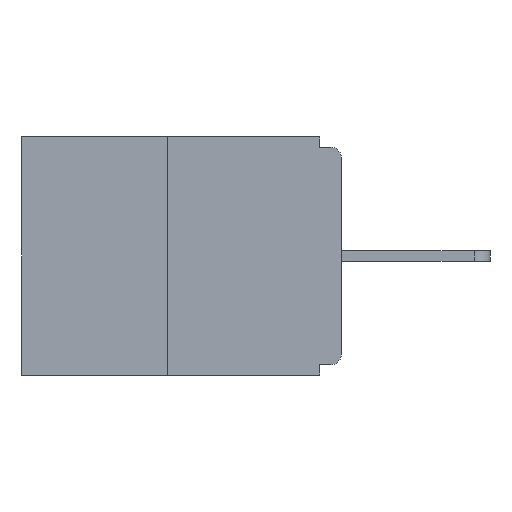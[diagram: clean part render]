
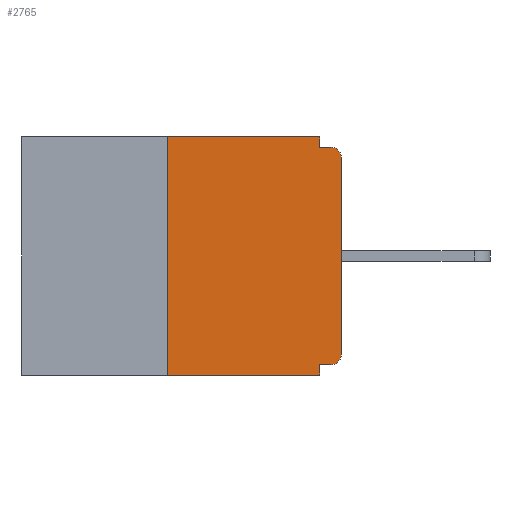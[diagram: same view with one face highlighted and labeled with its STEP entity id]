
A CAD part, left-side view. The second image highlights one B-rep face of the part: STEP entity #2765.
In plain terms, the highlighted planar face has unit normal (-1, 0, 0).
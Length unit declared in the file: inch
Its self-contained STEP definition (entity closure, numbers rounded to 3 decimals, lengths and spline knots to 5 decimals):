
#239 = EDGE_CURVE ( 'NONE', #16663, #10309, #5698, .T. ) ;
#665 = LINE ( 'NONE', #3332, #12376 ) ;
#744 = DIRECTION ( 'NONE',  ( 0., 1., 0. ) ) ;
#1418 = CARTESIAN_POINT ( 'NONE',  ( 0., 0.015, -0.015 ) ) ;
#1787 = DIRECTION ( 'NONE',  ( 0., -1., 0. ) ) ;
#1801 = ORIENTED_EDGE ( 'NONE', *, *, #16502, .F. ) ;
#2765 = ADVANCED_FACE ( 'NONE', ( #12053 ), #13118, .F. ) ;
#3188 = CARTESIAN_POINT ( 'NONE',  ( 0., 0., -0.015 ) ) ;
#3332 = CARTESIAN_POINT ( 'NONE',  ( 0., 0., 0. ) ) ;
#3457 = ORIENTED_EDGE ( 'NONE', *, *, #5095, .T. ) ;
#3521 = LINE ( 'NONE', #13514, #7980 ) ;
#3758 = CARTESIAN_POINT ( 'NONE',  ( 0., 0.46, -0.343 ) ) ;
#4011 = CARTESIAN_POINT ( 'NONE',  ( 0., 0.031, -0.343 ) ) ;
#4619 = ORIENTED_EDGE ( 'NONE', *, *, #11678, .F. ) ;
#4798 = CARTESIAN_POINT ( 'NONE',  ( 0., 0.46, 0. ) ) ;
#5000 = CARTESIAN_POINT ( 'NONE',  ( 0., 0., -0.313 ) ) ;
#5095 = EDGE_CURVE ( 'NONE', #15963, #8422, #14659, .T. ) ;
#5176 = DIRECTION ( 'NONE',  ( 0., 0., -1. ) ) ;
#5457 = EDGE_LOOP ( 'NONE', ( #1801, #9594, #7517, #4619, #17503, #3457, #9910, #11811, #14829, #15544 ) ) ;
#5698 = LINE ( 'NONE', #3758, #15821 ) ;
#5871 = EDGE_CURVE ( 'NONE', #8422, #12729, #665, .T. ) ;
#5959 = VECTOR ( 'NONE', #6125, 39.37008 ) ;
#6125 = DIRECTION ( 'NONE',  ( 0., -1., 0. ) ) ;
#6165 = DIRECTION ( 'NONE',  ( 1., 0., 0. ) ) ;
#6712 = AXIS2_PLACEMENT_3D ( 'NONE', #4798, #6165, #13174 ) ;
#6737 = VERTEX_POINT ( 'NONE', #17194 ) ;
#6806 = DIRECTION ( 'NONE',  ( -1., 0., 0. ) ) ;
#7517 = ORIENTED_EDGE ( 'NONE', *, *, #239, .T. ) ;
#7595 = CARTESIAN_POINT ( 'NONE',  ( 0., 0.015, -0.313 ) ) ;
#7692 = CARTESIAN_POINT ( 'NONE',  ( 0., 0.46, 0. ) ) ;
#7980 = VECTOR ( 'NONE', #9082, 39.37008 ) ;
#8422 = VERTEX_POINT ( 'NONE', #5000 ) ;
#8779 = DIRECTION ( 'NONE',  ( 0., 0., -1. ) ) ;
#9082 = DIRECTION ( 'NONE',  ( 0., 0., 1. ) ) ;
#9594 = ORIENTED_EDGE ( 'NONE', *, *, #18240, .F. ) ;
#9910 = ORIENTED_EDGE ( 'NONE', *, *, #5871, .T. ) ;
#10309 = VERTEX_POINT ( 'NONE', #4011 ) ;
#10701 = LINE ( 'NONE', #12587, #17488 ) ;
#10847 = LINE ( 'NONE', #7692, #11068 ) ;
#11066 = CARTESIAN_POINT ( 'NONE',  ( 0., 0.015, -0.03 ) ) ;
#11068 = VECTOR ( 'NONE', #1787, 39.37008 ) ;
#11678 = EDGE_CURVE ( 'NONE', #16918, #10309, #10701, .T. ) ;
#11811 = ORIENTED_EDGE ( 'NONE', *, *, #14059, .T. ) ;
#11889 = CARTESIAN_POINT ( 'NONE',  ( 0., 0.25, 0. ) ) ;
#12053 = FACE_OUTER_BOUND ( 'NONE', #5457, .T. ) ;
#12054 = LINE ( 'NONE', #16778, #12982 ) ;
#12376 = VECTOR ( 'NONE', #13469, 39.37008 ) ;
#12473 = VERTEX_POINT ( 'NONE', #1418 ) ;
#12587 = CARTESIAN_POINT ( 'NONE',  ( 0., 0.031, -0.343 ) ) ;
#12593 = EDGE_CURVE ( 'NONE', #6737, #12473, #12742, .T. ) ;
#12729 = VERTEX_POINT ( 'NONE', #14951 ) ;
#12742 = LINE ( 'NONE', #3188, #5959 ) ;
#12982 = VECTOR ( 'NONE', #5176, 39.37008 ) ;
#13118 = PLANE ( 'NONE',  #6712 ) ;
#13132 = CIRCLE ( 'NONE', #16156, 0.015 ) ;
#13174 = DIRECTION ( 'NONE',  ( 0., 0., -1. ) ) ;
#13469 = DIRECTION ( 'NONE',  ( 0., 0., 1. ) ) ;
#13514 = CARTESIAN_POINT ( 'NONE',  ( 0., 0.25, 0. ) ) ;
#14059 = EDGE_CURVE ( 'NONE', #12729, #12473, #13132, .T. ) ;
#14097 = DIRECTION ( 'NONE',  ( 0., 0., -1. ) ) ;
#14659 = CIRCLE ( 'NONE', #18574, 0.015 ) ;
#14731 = CARTESIAN_POINT ( 'NONE',  ( 0., 0.031, 0. ) ) ;
#14829 = ORIENTED_EDGE ( 'NONE', *, *, #12593, .F. ) ;
#14951 = CARTESIAN_POINT ( 'NONE',  ( 0., 0., -0.03 ) ) ;
#15544 = ORIENTED_EDGE ( 'NONE', *, *, #17888, .F. ) ;
#15821 = VECTOR ( 'NONE', #16677, 39.37008 ) ;
#15963 = VERTEX_POINT ( 'NONE', #18510 ) ;
#16060 = CARTESIAN_POINT ( 'NONE',  ( 0., 0.031, -0.328 ) ) ;
#16156 = AXIS2_PLACEMENT_3D ( 'NONE', #11066, #6806, #18393 ) ;
#16483 = LINE ( 'NONE', #17970, #17399 ) ;
#16502 = EDGE_CURVE ( 'NONE', #16819, #17355, #10847, .T. ) ;
#16663 = VERTEX_POINT ( 'NONE', #17885 ) ;
#16677 = DIRECTION ( 'NONE',  ( 0., -1., 0. ) ) ;
#16778 = CARTESIAN_POINT ( 'NONE',  ( 0., 0.031, 0. ) ) ;
#16819 = VERTEX_POINT ( 'NONE', #11889 ) ;
#16918 = VERTEX_POINT ( 'NONE', #16060 ) ;
#17194 = CARTESIAN_POINT ( 'NONE',  ( 0., 0.031, -0.015 ) ) ;
#17355 = VERTEX_POINT ( 'NONE', #14731 ) ;
#17399 = VECTOR ( 'NONE', #744, 39.37008 ) ;
#17487 = EDGE_CURVE ( 'NONE', #15963, #16918, #16483, .T. ) ;
#17488 = VECTOR ( 'NONE', #14097, 39.37008 ) ;
#17503 = ORIENTED_EDGE ( 'NONE', *, *, #17487, .F. ) ;
#17669 = DIRECTION ( 'NONE',  ( -1., 0., 0. ) ) ;
#17885 = CARTESIAN_POINT ( 'NONE',  ( 0., 0.25, -0.343 ) ) ;
#17888 = EDGE_CURVE ( 'NONE', #17355, #6737, #12054, .T. ) ;
#17970 = CARTESIAN_POINT ( 'NONE',  ( 0., 0., -0.328 ) ) ;
#18240 = EDGE_CURVE ( 'NONE', #16663, #16819, #3521, .T. ) ;
#18393 = DIRECTION ( 'NONE',  ( 0., 0., -1. ) ) ;
#18510 = CARTESIAN_POINT ( 'NONE',  ( 0., 0.015, -0.328 ) ) ;
#18574 = AXIS2_PLACEMENT_3D ( 'NONE', #7595, #17669, #8779 ) ;
